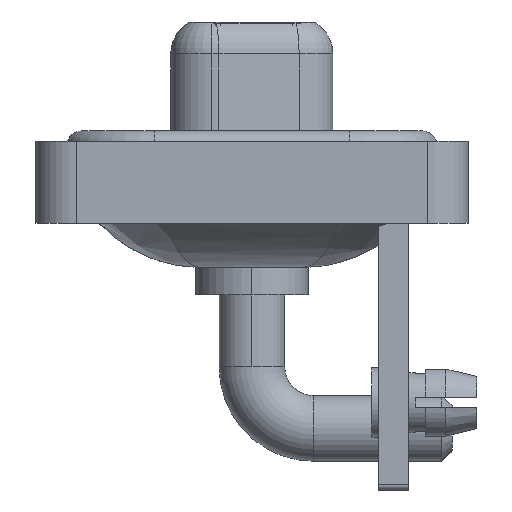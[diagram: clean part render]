
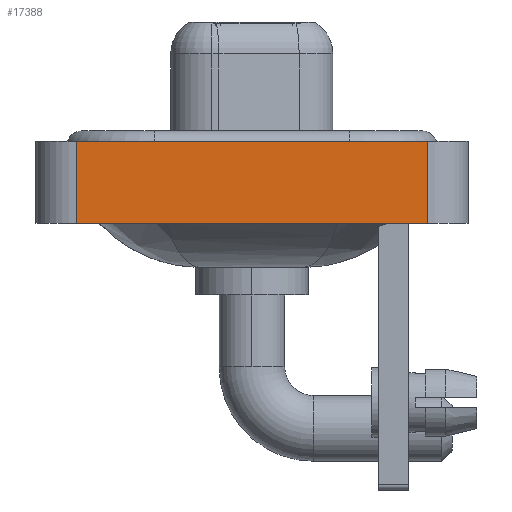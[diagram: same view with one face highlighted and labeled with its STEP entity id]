
A CAD part, left-side view. The second image highlights one B-rep face of the part: STEP entity #17388.
In plain terms, the highlighted planar face has unit normal (-1, 0, 0).
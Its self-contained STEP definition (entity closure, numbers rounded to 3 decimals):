
#140 = CARTESIAN_POINT ( 'NONE',  ( -7.25, 8.55, -3.6 ) ) ;
#566 = PLANE ( 'NONE',  #12026 ) ;
#967 = EDGE_LOOP ( 'NONE', ( #15907, #2135, #14817, #14589 ) ) ;
#1082 = VERTEX_POINT ( 'NONE', #10468 ) ;
#2135 = ORIENTED_EDGE ( 'NONE', *, *, #5260, .F. ) ;
#2296 = CARTESIAN_POINT ( 'NONE',  ( -7.25, -8.55, 0.4 ) ) ;
#2735 = EDGE_CURVE ( 'NONE', #4748, #13258, #10191, .T. ) ;
#3290 = VECTOR ( 'NONE', #9908, 1000. ) ;
#4748 = VERTEX_POINT ( 'NONE', #15836 ) ;
#5260 = EDGE_CURVE ( 'NONE', #15346, #13258, #7339, .T. ) ;
#6065 = CARTESIAN_POINT ( 'NONE',  ( -7.25, -8.55, 0.4 ) ) ;
#6769 = CARTESIAN_POINT ( 'NONE',  ( -7.25, -8.55, -3.6 ) ) ;
#7290 = CARTESIAN_POINT ( 'NONE',  ( -7.25, -8.55, -3.6 ) ) ;
#7339 = LINE ( 'NONE', #6065, #10131 ) ;
#7527 = DIRECTION ( 'NONE',  ( 0., -1., 0. ) ) ;
#8846 = DIRECTION ( 'NONE',  ( 0., 0., 1. ) ) ;
#9908 = DIRECTION ( 'NONE',  ( 0., 0., 1. ) ) ;
#10131 = VECTOR ( 'NONE', #7527, 1000. ) ;
#10191 = LINE ( 'NONE', #16818, #3290 ) ;
#10468 = CARTESIAN_POINT ( 'NONE',  ( -7.25, 8.55, -3.6 ) ) ;
#11747 = DIRECTION ( 'NONE',  ( 0., 0., 1. ) ) ;
#12026 = AXIS2_PLACEMENT_3D ( 'NONE', #7290, #12905, #8846 ) ;
#12300 = DIRECTION ( 'NONE',  ( 0., -1., 0. ) ) ;
#12356 = VECTOR ( 'NONE', #12300, 1000. ) ;
#12905 = DIRECTION ( 'NONE',  ( -1., 0., 0. ) ) ;
#13258 = VERTEX_POINT ( 'NONE', #2296 ) ;
#13935 = LINE ( 'NONE', #6769, #12356 ) ;
#14298 = FACE_OUTER_BOUND ( 'NONE', #967, .T. ) ;
#14508 = CARTESIAN_POINT ( 'NONE',  ( -7.25, 8.55, 0.4 ) ) ;
#14589 = ORIENTED_EDGE ( 'NONE', *, *, #15625, .T. ) ;
#14817 = ORIENTED_EDGE ( 'NONE', *, *, #16768, .F. ) ;
#15346 = VERTEX_POINT ( 'NONE', #14508 ) ;
#15625 = EDGE_CURVE ( 'NONE', #1082, #4748, #13935, .T. ) ;
#15700 = LINE ( 'NONE', #140, #16159 ) ;
#15836 = CARTESIAN_POINT ( 'NONE',  ( -7.25, -8.55, -3.6 ) ) ;
#15907 = ORIENTED_EDGE ( 'NONE', *, *, #2735, .T. ) ;
#16159 = VECTOR ( 'NONE', #11747, 1000. ) ;
#16768 = EDGE_CURVE ( 'NONE', #1082, #15346, #15700, .T. ) ;
#16818 = CARTESIAN_POINT ( 'NONE',  ( -7.25, -8.55, -3.6 ) ) ;
#17388 = ADVANCED_FACE ( 'NONE', ( #14298 ), #566, .T. ) ;
